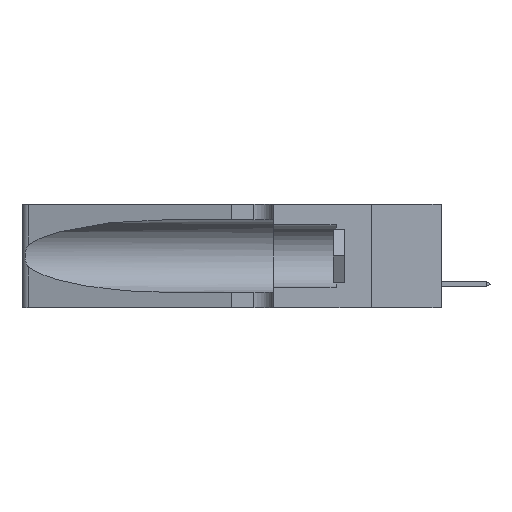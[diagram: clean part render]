
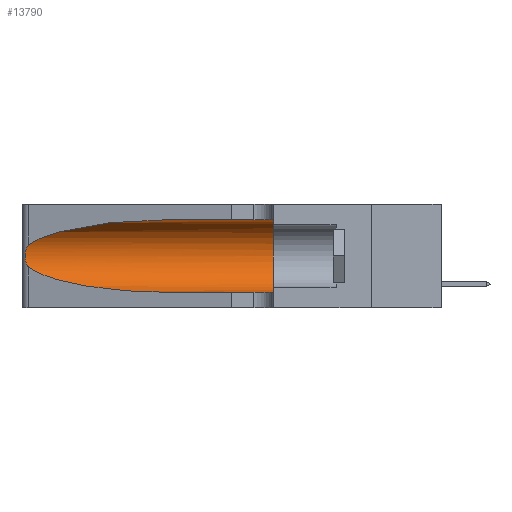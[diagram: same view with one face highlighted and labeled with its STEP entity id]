
A CAD part, left-side view. The second image highlights one B-rep face of the part: STEP entity #13790.
In plain terms, the highlighted cylindrical face has radius 3.308 mm (diameter 6.617 mm), a partial arc.
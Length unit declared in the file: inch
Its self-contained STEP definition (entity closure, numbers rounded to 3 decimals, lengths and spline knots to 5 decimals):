
#1371 = DIRECTION ( 'NONE',  ( 0., -1., 0. ) ) ;
#1908 = CARTESIAN_POINT ( 'NONE',  ( 0.25487, 1.22718, 0.14631 ) ) ;
#2287 = CARTESIAN_POINT ( 'NONE',  ( 0.25639, 1.23184, 0.21858 ) ) ;
#2598 = CARTESIAN_POINT ( 'NONE',  ( 0.25787, 1.23484, 0.2124 ) ) ;
#3569 = B_SPLINE_CURVE_WITH_KNOTS ( 'NONE', 3,
 ( #27889, #15832, #2287, #2598, #5729, #5874, #41766, #5438, #22104, #28921, #25298, #38788, #8635, #15221 ),
 .UNSPECIFIED., .F., .F.,
 ( 4, 2, 2, 2, 2, 2, 4 ),
 ( 0., 0.00027, 0.00053, 0.00107, 0.0016, 0.00187, 0.00214 ),
 .UNSPECIFIED. ) ;
#5280 = EDGE_CURVE ( 'NONE', #10537, #39096, #22791, .T. ) ;
#5420 = CYLINDRICAL_SURFACE ( 'NONE', #8435, 0.13025 ) ;
#5438 = CARTESIAN_POINT ( 'NONE',  ( 0.26075, 1.23896, 0.178 ) ) ;
#5729 = CARTESIAN_POINT ( 'NONE',  ( 0.25854, 1.2359, 0.20912 ) ) ;
#5874 = CARTESIAN_POINT ( 'NONE',  ( 0.26018, 1.23835, 0.19895 ) ) ;
#6344 = CARTESIAN_POINT ( 'NONE',  ( 0.25487, 1.22718, 0.22369 ) ) ;
#7758 = CARTESIAN_POINT ( 'NONE',  ( 0.18966, 0.96281, 0.31525 ) ) ;
#8368 = CARTESIAN_POINT ( 'NONE',  ( 0.1305, 0.72297, 0.31525 ) ) ;
#8435 = AXIS2_PLACEMENT_3D ( 'NONE', #19951, #40613, #30869 ) ;
#8635 = CARTESIAN_POINT ( 'NONE',  ( 0.25555, 1.22993, 0.14849 ) ) ;
#9126 = CARTESIAN_POINT ( 'NONE',  ( 0.1305, 1.61858, 0.05475 ) ) ;
#9980 = DIRECTION ( 'NONE',  ( 0., 0., 1. ) ) ;
#10143 = CARTESIAN_POINT ( 'NONE',  ( 0.1305, 0.35, 0.31525 ) ) ;
#10537 = VERTEX_POINT ( 'NONE', #24190 ) ;
#10596 = VERTEX_POINT ( 'NONE', #14422 ) ;
#10936 = AXIS2_PLACEMENT_3D ( 'NONE', #23444, #23311, #9980 ) ;
#11905 = CARTESIAN_POINT ( 'NONE',  ( 0.1305, 0.72297, 0.05475 ) ) ;
#12411 = DIRECTION ( 'NONE',  ( 0., -1., 0. ) ) ;
#13790 = ADVANCED_FACE ( 'NONE', ( #16468 ), #5420, .F. ) ;
#14422 = CARTESIAN_POINT ( 'NONE',  ( 0.1305, 0.35, 0.05475 ) ) ;
#15221 = CARTESIAN_POINT ( 'NONE',  ( 0.25487, 1.22718, 0.14631 ) ) ;
#15832 = CARTESIAN_POINT ( 'NONE',  ( 0.25555, 1.22994, 0.2215 ) ) ;
#16468 = FACE_OUTER_BOUND ( 'NONE', #23114, .T. ) ;
#16495 = LINE ( 'NONE', #28150, #17965 ) ;
#17965 = VECTOR ( 'NONE', #1371, 39.37008 ) ;
#18805 = EDGE_CURVE ( 'NONE', #10537, #33499, #16495, .T. ) ;
#19452 = VERTEX_POINT ( 'NONE', #11905 ) ;
#19556 = CARTESIAN_POINT ( 'NONE',  ( 0.18966, 0.96281, 0.05475 ) ) ;
#19951 = CARTESIAN_POINT ( 'NONE',  ( 0.1305, 1.61858, 0.185 ) ) ;
#21243 = VERTEX_POINT ( 'NONE', #1908 ) ;
#21969 = ORIENTED_EDGE ( 'NONE', *, *, #5280, .T. ) ;
#22104 = CARTESIAN_POINT ( 'NONE',  ( 0.26017, 1.23833, 0.17102 ) ) ;
#22111 = CIRCLE ( 'NONE', #10936, 0.13025 ) ;
#22285 = EDGE_CURVE ( 'NONE', #19452, #10596, #31236, .T. ) ;
#22606 = CARTESIAN_POINT ( 'NONE',  ( 0.25487, 1.22718, 0.14631 ) ) ;
#22791 =( BOUNDED_CURVE ( )  B_SPLINE_CURVE ( 3, ( #8368, #7758, #34043, #40648 ),
 .UNSPECIFIED., .F., .F. ) 
 B_SPLINE_CURVE_WITH_KNOTS ( ( 4, 4 ),
 ( 1.5708, 2.84003 ),
 .UNSPECIFIED. ) 
 CURVE ( )  GEOMETRIC_REPRESENTATION_ITEM ( )  RATIONAL_B_SPLINE_CURVE ( ( 1., 0.87, 0.87, 1. ) ) 
 REPRESENTATION_ITEM ( '' )  );
#23114 = EDGE_LOOP ( 'NONE', ( #21969, #40324, #42074, #35322, #39643, #33020 ) ) ;
#23311 = DIRECTION ( 'NONE',  ( 0., 1., 0. ) ) ;
#23444 = CARTESIAN_POINT ( 'NONE',  ( 0.1305, 0.35, 0.185 ) ) ;
#24190 = CARTESIAN_POINT ( 'NONE',  ( 0.1305, 0.72297, 0.31525 ) ) ;
#25298 = CARTESIAN_POINT ( 'NONE',  ( 0.25789, 1.23486, 0.15765 ) ) ;
#26634 = VECTOR ( 'NONE', #12411, 39.37008 ) ;
#27715 = EDGE_CURVE ( 'NONE', #39096, #21243, #3569, .T. ) ;
#27889 = CARTESIAN_POINT ( 'NONE',  ( 0.25487, 1.22718, 0.22369 ) ) ;
#28150 = CARTESIAN_POINT ( 'NONE',  ( 0.1305, 1.61858, 0.31525 ) ) ;
#28349 =( BOUNDED_CURVE ( )  B_SPLINE_CURVE ( 3, ( #22606, #39369, #19556, #32650 ),
 .UNSPECIFIED., .F., .T. ) 
 B_SPLINE_CURVE_WITH_KNOTS ( ( 4, 4 ),
 ( 3.44316, 4.71239 ),
 .UNSPECIFIED. ) 
 CURVE ( )  GEOMETRIC_REPRESENTATION_ITEM ( )  RATIONAL_B_SPLINE_CURVE ( ( 1., 0.87, 0.87, 1. ) ) 
 REPRESENTATION_ITEM ( '' )  );
#28921 = CARTESIAN_POINT ( 'NONE',  ( 0.25856, 1.23593, 0.16098 ) ) ;
#30869 = DIRECTION ( 'NONE',  ( 0., 0., -1. ) ) ;
#31236 = LINE ( 'NONE', #9126, #26634 ) ;
#32650 = CARTESIAN_POINT ( 'NONE',  ( 0.1305, 0.72297, 0.05475 ) ) ;
#33020 = ORIENTED_EDGE ( 'NONE', *, *, #18805, .F. ) ;
#33499 = VERTEX_POINT ( 'NONE', #10143 ) ;
#34043 = CARTESIAN_POINT ( 'NONE',  ( 0.2373, 1.15595, 0.28018 ) ) ;
#34700 = EDGE_CURVE ( 'NONE', #21243, #19452, #28349, .T. ) ;
#35322 = ORIENTED_EDGE ( 'NONE', *, *, #22285, .T. ) ;
#38788 = CARTESIAN_POINT ( 'NONE',  ( 0.25639, 1.23186, 0.15144 ) ) ;
#39096 = VERTEX_POINT ( 'NONE', #6344 ) ;
#39369 = CARTESIAN_POINT ( 'NONE',  ( 0.2373, 1.15595, 0.08982 ) ) ;
#39643 = ORIENTED_EDGE ( 'NONE', *, *, #42038, .F. ) ;
#40324 = ORIENTED_EDGE ( 'NONE', *, *, #27715, .T. ) ;
#40613 = DIRECTION ( 'NONE',  ( 0., -1., 0. ) ) ;
#40648 = CARTESIAN_POINT ( 'NONE',  ( 0.25487, 1.22718, 0.22369 ) ) ;
#41766 = CARTESIAN_POINT ( 'NONE',  ( 0.26075, 1.23896, 0.19203 ) ) ;
#42038 = EDGE_CURVE ( 'NONE', #33499, #10596, #22111, .T. ) ;
#42074 = ORIENTED_EDGE ( 'NONE', *, *, #34700, .T. ) ;
